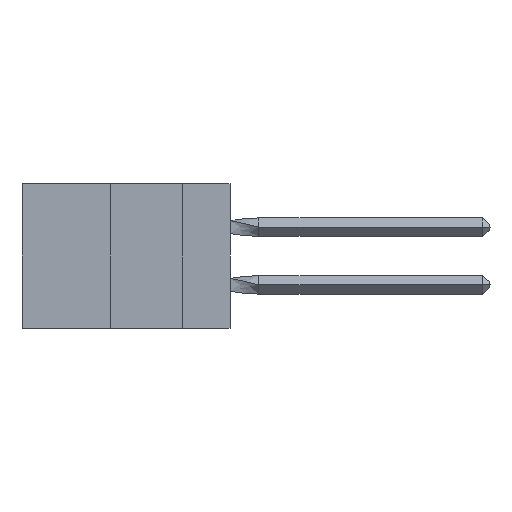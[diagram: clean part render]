
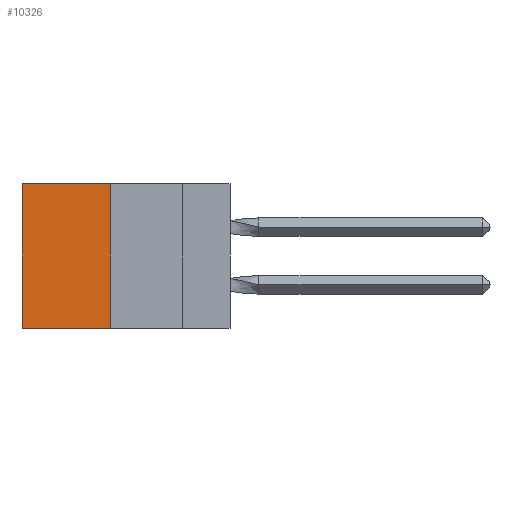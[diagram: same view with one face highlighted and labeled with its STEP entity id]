
A CAD part, left-side view. The second image highlights one B-rep face of the part: STEP entity #10326.
In plain terms, the highlighted planar face has unit normal (-1, 0, 0).
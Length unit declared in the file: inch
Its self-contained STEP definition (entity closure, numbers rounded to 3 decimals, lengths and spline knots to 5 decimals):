
#1 = DIRECTION ( 'NONE',  ( 0., 0., -1. ) ) ;
#158 = EDGE_LOOP ( 'NONE', ( #8458, #3250, #7608, #13171 ) ) ;
#658 = VERTEX_POINT ( 'NONE', #11430 ) ;
#1431 = DIRECTION ( 'NONE',  ( 0., 1., 0. ) ) ;
#1658 = DIRECTION ( 'NONE',  ( 1., 0., 0. ) ) ;
#1722 = PLANE ( 'NONE',  #9106 ) ;
#2068 = EDGE_CURVE ( 'NONE', #8169, #7451, #16633, .T. ) ;
#2085 = EDGE_CURVE ( 'NONE', #658, #6799, #12000, .T. ) ;
#2218 = EDGE_CURVE ( 'NONE', #658, #8169, #17615, .T. ) ;
#2242 = VECTOR ( 'NONE', #6571, 39.37008 ) ;
#2747 = VECTOR ( 'NONE', #1431, 39.37008 ) ;
#3250 = ORIENTED_EDGE ( 'NONE', *, *, #2068, .F. ) ;
#3506 = DIRECTION ( 'NONE',  ( 0., 0., -1. ) ) ;
#5833 = EDGE_CURVE ( 'NONE', #6799, #7451, #6420, .T. ) ;
#6420 = LINE ( 'NONE', #12994, #2242 ) ;
#6571 = DIRECTION ( 'NONE',  ( 0., 0., -1. ) ) ;
#6799 = VERTEX_POINT ( 'NONE', #7840 ) ;
#7451 = VERTEX_POINT ( 'NONE', #18285 ) ;
#7608 = ORIENTED_EDGE ( 'NONE', *, *, #2218, .F. ) ;
#7795 = CARTESIAN_POINT ( 'NONE',  ( 0.305, 0.413, -0.5 ) ) ;
#7840 = CARTESIAN_POINT ( 'NONE',  ( 0.305, 0.72, 0. ) ) ;
#8169 = VERTEX_POINT ( 'NONE', #15288 ) ;
#8354 = VECTOR ( 'NONE', #3506, 39.37008 ) ;
#8458 = ORIENTED_EDGE ( 'NONE', *, *, #5833, .T. ) ;
#9106 = AXIS2_PLACEMENT_3D ( 'NONE', #15563, #1658, #1 ) ;
#10326 = ADVANCED_FACE ( 'NONE', ( #15694 ), #1722, .F. ) ;
#11430 = CARTESIAN_POINT ( 'NONE',  ( 0.305, 0.413, 0. ) ) ;
#12000 = LINE ( 'NONE', #17033, #2747 ) ;
#12495 = VECTOR ( 'NONE', #12554, 39.37008 ) ;
#12554 = DIRECTION ( 'NONE',  ( 0., 1., 0. ) ) ;
#12994 = CARTESIAN_POINT ( 'NONE',  ( 0.305, 0.72, -0.5 ) ) ;
#13171 = ORIENTED_EDGE ( 'NONE', *, *, #2085, .T. ) ;
#15288 = CARTESIAN_POINT ( 'NONE',  ( 0.305, 0.413, -0.5 ) ) ;
#15563 = CARTESIAN_POINT ( 'NONE',  ( 0.305, 0.413, -0.5 ) ) ;
#15694 = FACE_OUTER_BOUND ( 'NONE', #158, .T. ) ;
#15815 = CARTESIAN_POINT ( 'NONE',  ( 0.305, 0.413, -0.5 ) ) ;
#16633 = LINE ( 'NONE', #7795, #12495 ) ;
#17033 = CARTESIAN_POINT ( 'NONE',  ( 0.305, 0.413, 0. ) ) ;
#17615 = LINE ( 'NONE', #15815, #8354 ) ;
#18285 = CARTESIAN_POINT ( 'NONE',  ( 0.305, 0.72, -0.5 ) ) ;
